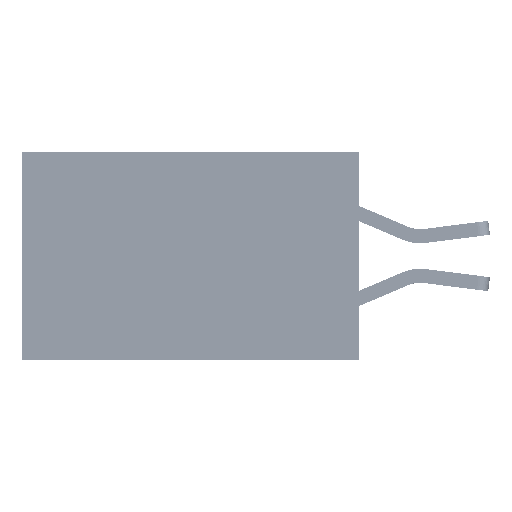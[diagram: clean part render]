
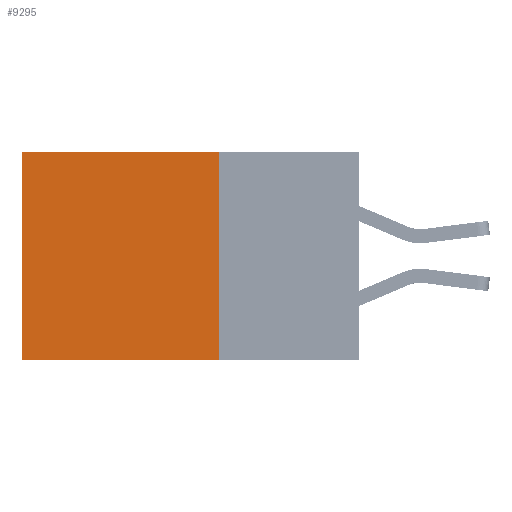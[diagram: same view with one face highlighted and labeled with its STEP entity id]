
A CAD part, left-side view. The second image highlights one B-rep face of the part: STEP entity #9295.
In plain terms, the highlighted planar face has unit normal (-1, 0, 0).
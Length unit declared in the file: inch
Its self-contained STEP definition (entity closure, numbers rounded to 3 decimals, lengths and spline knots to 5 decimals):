
#820 = CARTESIAN_POINT ( 'NONE',  ( 0.2875, 0.6, 0. ) ) ;
#1205 = CARTESIAN_POINT ( 'NONE',  ( 0.2875, 0.25, 0. ) ) ;
#2716 = VECTOR ( 'NONE', #5081, 39.37008 ) ;
#3189 = CARTESIAN_POINT ( 'NONE',  ( 0.2875, 0.25, 0. ) ) ;
#3207 = CARTESIAN_POINT ( 'NONE',  ( 0.2875, 0.25, -0.37 ) ) ;
#3872 = LINE ( 'NONE', #1205, #2716 ) ;
#4371 = DIRECTION ( 'NONE',  ( 0., 0., -1. ) ) ;
#5081 = DIRECTION ( 'NONE',  ( 0., 1., 0. ) ) ;
#6589 = EDGE_CURVE ( 'NONE', #26086, #32732, #3872, .T. ) ;
#9295 = ADVANCED_FACE ( 'NONE', ( #35752 ), #28760, .F. ) ;
#9442 = VERTEX_POINT ( 'NONE', #41073 ) ;
#9468 = ORIENTED_EDGE ( 'NONE', *, *, #31209, .F. ) ;
#10289 = VERTEX_POINT ( 'NONE', #27398 ) ;
#17019 = ORIENTED_EDGE ( 'NONE', *, *, #6589, .T. ) ;
#17155 = ORIENTED_EDGE ( 'NONE', *, *, #44427, .T. ) ;
#21385 = DIRECTION ( 'NONE',  ( 0., 1., 0. ) ) ;
#21685 = DIRECTION ( 'NONE',  ( 0., 0., -1. ) ) ;
#22829 = LINE ( 'NONE', #3207, #41174 ) ;
#23137 = VECTOR ( 'NONE', #34552, 39.37008 ) ;
#26086 = VERTEX_POINT ( 'NONE', #28399 ) ;
#27398 = CARTESIAN_POINT ( 'NONE',  ( 0.2875, 0.6, -0.37 ) ) ;
#28399 = CARTESIAN_POINT ( 'NONE',  ( 0.2875, 0.25, 0. ) ) ;
#28760 = PLANE ( 'NONE',  #40034 ) ;
#29443 = LINE ( 'NONE', #30567, #23137 ) ;
#30105 = CARTESIAN_POINT ( 'NONE',  ( 0.2875, 0.6, 0. ) ) ;
#30567 = CARTESIAN_POINT ( 'NONE',  ( 0.2875, 0.25, 0. ) ) ;
#31209 = EDGE_CURVE ( 'NONE', #9442, #10289, #22829, .T. ) ;
#31642 = ORIENTED_EDGE ( 'NONE', *, *, #36428, .F. ) ;
#31961 = EDGE_LOOP ( 'NONE', ( #17155, #9468, #31642, #17019 ) ) ;
#32158 = LINE ( 'NONE', #820, #37344 ) ;
#32732 = VERTEX_POINT ( 'NONE', #30105 ) ;
#34552 = DIRECTION ( 'NONE',  ( 0., 0., -1. ) ) ;
#35752 = FACE_OUTER_BOUND ( 'NONE', #31961, .T. ) ;
#36306 = DIRECTION ( 'NONE',  ( 1., 0., 0. ) ) ;
#36428 = EDGE_CURVE ( 'NONE', #26086, #9442, #29443, .T. ) ;
#37344 = VECTOR ( 'NONE', #4371, 39.37008 ) ;
#40034 = AXIS2_PLACEMENT_3D ( 'NONE', #3189, #36306, #21685 ) ;
#41073 = CARTESIAN_POINT ( 'NONE',  ( 0.2875, 0.25, -0.37 ) ) ;
#41174 = VECTOR ( 'NONE', #21385, 39.37008 ) ;
#44427 = EDGE_CURVE ( 'NONE', #32732, #10289, #32158, .T. ) ;
